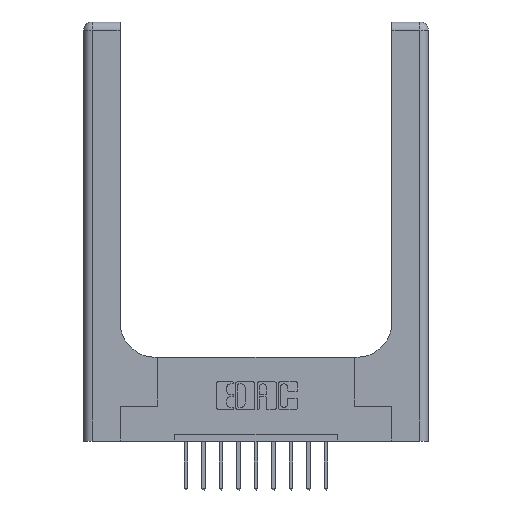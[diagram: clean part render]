
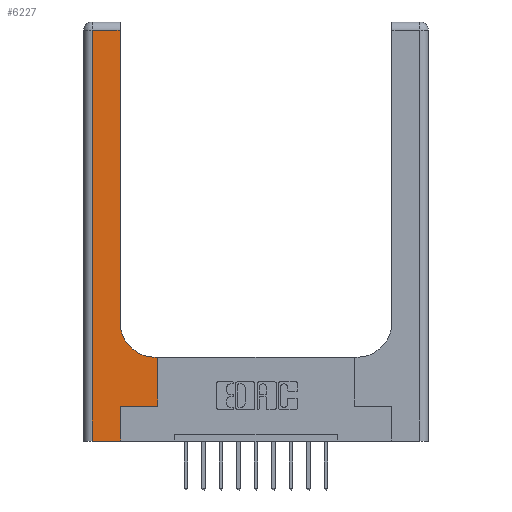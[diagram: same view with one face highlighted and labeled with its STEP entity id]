
A CAD part, top view. The second image highlights one B-rep face of the part: STEP entity #6227.
In plain terms, the highlighted planar face has unit normal (0, 0, 1).
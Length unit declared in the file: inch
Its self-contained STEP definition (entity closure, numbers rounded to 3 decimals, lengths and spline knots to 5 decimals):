
#59 = EDGE_LOOP ( 'NONE', ( #7840, #5813, #11852, #2579, #687, #9921, #979, #15053, #1505 ) ) ;
#152 = LINE ( 'NONE', #1416, #1819 ) ;
#192 = VERTEX_POINT ( 'NONE', #7194 ) ;
#687 = ORIENTED_EDGE ( 'NONE', *, *, #11968, .T. ) ;
#735 = PLANE ( 'NONE',  #6273 ) ;
#845 = CARTESIAN_POINT ( 'NONE',  ( 0.528, 0.25, 0.37 ) ) ;
#851 = CARTESIAN_POINT ( 'NONE',  ( 0.51, 0.85, 0.37 ) ) ;
#979 = ORIENTED_EDGE ( 'NONE', *, *, #12505, .T. ) ;
#1021 = VERTEX_POINT ( 'NONE', #7137 ) ;
#1046 = EDGE_CURVE ( 'NONE', #10355, #14236, #3626, .T. ) ;
#1322 = VECTOR ( 'NONE', #7902, 39.37008 ) ;
#1372 = CARTESIAN_POINT ( 'NONE',  ( 0.06, 2.94, 0.37 ) ) ;
#1416 = CARTESIAN_POINT ( 'NONE',  ( 0.265, 0., 0.37 ) ) ;
#1505 = ORIENTED_EDGE ( 'NONE', *, *, #11050, .T. ) ;
#1510 = DIRECTION ( 'NONE',  ( 1., 0., 0. ) ) ;
#1745 = CARTESIAN_POINT ( 'NONE',  ( 0.528, 0.6, 0.37 ) ) ;
#1819 = VECTOR ( 'NONE', #14900, 39.37008 ) ;
#1851 = EDGE_CURVE ( 'NONE', #7073, #1021, #2506, .T. ) ;
#2269 = CARTESIAN_POINT ( 'NONE',  ( 0., 0., 0.37 ) ) ;
#2275 = VERTEX_POINT ( 'NONE', #1372 ) ;
#2506 = LINE ( 'NONE', #7503, #9211 ) ;
#2579 = ORIENTED_EDGE ( 'NONE', *, *, #8473, .T. ) ;
#2710 = LINE ( 'NONE', #7556, #14771 ) ;
#3131 = LINE ( 'NONE', #2269, #8313 ) ;
#3511 = LINE ( 'NONE', #7176, #12746 ) ;
#3561 = EDGE_CURVE ( 'NONE', #2275, #6033, #4211, .T. ) ;
#3626 = LINE ( 'NONE', #3704, #7109 ) ;
#3704 = CARTESIAN_POINT ( 'NONE',  ( 0.265, 0.25, 0.37 ) ) ;
#3728 = DIRECTION ( 'NONE',  ( 0., 0., -1. ) ) ;
#3955 = DIRECTION ( 'NONE',  ( -1., 0., 0. ) ) ;
#4152 = LINE ( 'NONE', #9159, #1322 ) ;
#4211 = LINE ( 'NONE', #8829, #11209 ) ;
#4937 = DIRECTION ( 'NONE',  ( 0., 1., 0. ) ) ;
#5671 = DIRECTION ( 'NONE',  ( 1., 0., 0. ) ) ;
#5813 = ORIENTED_EDGE ( 'NONE', *, *, #14947, .T. ) ;
#5821 = CARTESIAN_POINT ( 'NONE',  ( 0.06, 0., 0.37 ) ) ;
#6033 = VERTEX_POINT ( 'NONE', #5821 ) ;
#6090 = AXIS2_PLACEMENT_3D ( 'NONE', #851, #3728, #5671 ) ;
#6227 = ADVANCED_FACE ( 'NONE', ( #9948 ), #735, .F. ) ;
#6273 = AXIS2_PLACEMENT_3D ( 'NONE', #15013, #8979, #13824 ) ;
#6532 = DIRECTION ( 'NONE',  ( 0., -1., 0. ) ) ;
#6585 = VERTEX_POINT ( 'NONE', #12483 ) ;
#6610 = CIRCLE ( 'NONE', #6090, 0.25 ) ;
#7073 = VERTEX_POINT ( 'NONE', #1745 ) ;
#7109 = VECTOR ( 'NONE', #1510, 39.37008 ) ;
#7137 = CARTESIAN_POINT ( 'NONE',  ( 0.51, 0.6, 0.37 ) ) ;
#7176 = CARTESIAN_POINT ( 'NONE',  ( 0.26, 3., 0.37 ) ) ;
#7194 = CARTESIAN_POINT ( 'NONE',  ( 0.26, 2.94, 0.37 ) ) ;
#7304 = VERTEX_POINT ( 'NONE', #11307 ) ;
#7503 = CARTESIAN_POINT ( 'NONE',  ( 0.26, 0.6, 0.37 ) ) ;
#7556 = CARTESIAN_POINT ( 'NONE',  ( 0., 2.94, 0.37 ) ) ;
#7840 = ORIENTED_EDGE ( 'NONE', *, *, #14353, .T. ) ;
#7902 = DIRECTION ( 'NONE',  ( 0., 1., 0. ) ) ;
#8313 = VECTOR ( 'NONE', #15336, 39.37008 ) ;
#8473 = EDGE_CURVE ( 'NONE', #6033, #7304, #3131, .T. ) ;
#8829 = CARTESIAN_POINT ( 'NONE',  ( 0.06, 3., 0.37 ) ) ;
#8979 = DIRECTION ( 'NONE',  ( 0., 0., -1. ) ) ;
#9159 = CARTESIAN_POINT ( 'NONE',  ( 0.528, 0.25, 0.37 ) ) ;
#9211 = VECTOR ( 'NONE', #12097, 39.37008 ) ;
#9921 = ORIENTED_EDGE ( 'NONE', *, *, #1046, .T. ) ;
#9948 = FACE_OUTER_BOUND ( 'NONE', #59, .T. ) ;
#10077 = CARTESIAN_POINT ( 'NONE',  ( 0.265, 0.25, 0.37 ) ) ;
#10355 = VERTEX_POINT ( 'NONE', #10077 ) ;
#11050 = EDGE_CURVE ( 'NONE', #1021, #6585, #6610, .T. ) ;
#11209 = VECTOR ( 'NONE', #6532, 39.37008 ) ;
#11307 = CARTESIAN_POINT ( 'NONE',  ( 0.265, 0., 0.37 ) ) ;
#11852 = ORIENTED_EDGE ( 'NONE', *, *, #3561, .T. ) ;
#11968 = EDGE_CURVE ( 'NONE', #7304, #10355, #152, .T. ) ;
#12097 = DIRECTION ( 'NONE',  ( -1., 0., 0. ) ) ;
#12483 = CARTESIAN_POINT ( 'NONE',  ( 0.26, 0.85, 0.37 ) ) ;
#12505 = EDGE_CURVE ( 'NONE', #14236, #7073, #4152, .T. ) ;
#12746 = VECTOR ( 'NONE', #4937, 39.37008 ) ;
#13824 = DIRECTION ( 'NONE',  ( -1., 0., 0. ) ) ;
#14236 = VERTEX_POINT ( 'NONE', #845 ) ;
#14353 = EDGE_CURVE ( 'NONE', #6585, #192, #3511, .T. ) ;
#14771 = VECTOR ( 'NONE', #3955, 39.37008 ) ;
#14900 = DIRECTION ( 'NONE',  ( 0., 1., 0. ) ) ;
#14947 = EDGE_CURVE ( 'NONE', #192, #2275, #2710, .T. ) ;
#15013 = CARTESIAN_POINT ( 'NONE',  ( 0., 3., 0.37 ) ) ;
#15053 = ORIENTED_EDGE ( 'NONE', *, *, #1851, .T. ) ;
#15336 = DIRECTION ( 'NONE',  ( 1., 0., 0. ) ) ;
